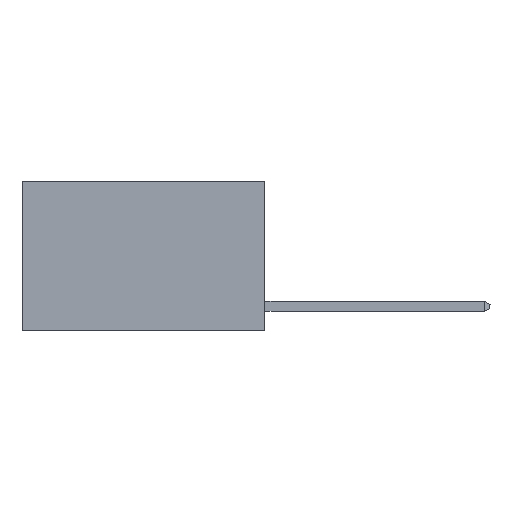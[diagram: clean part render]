
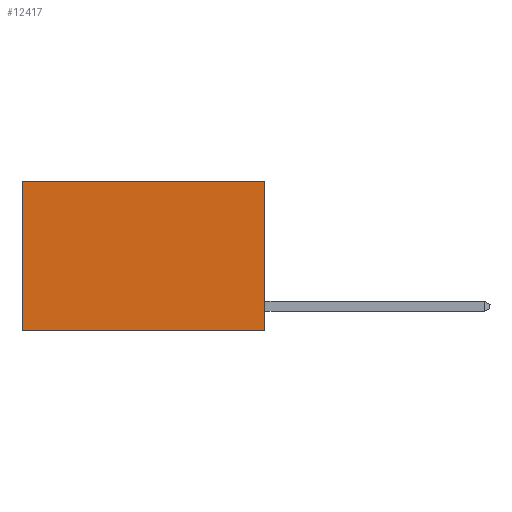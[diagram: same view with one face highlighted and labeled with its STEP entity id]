
A CAD part, left-side view. The second image highlights one B-rep face of the part: STEP entity #12417.
In plain terms, the highlighted planar face has unit normal (-1, 0, 0).
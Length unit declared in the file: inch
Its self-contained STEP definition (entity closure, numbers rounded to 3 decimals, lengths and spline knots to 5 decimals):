
#663 = CARTESIAN_POINT ( 'NONE',  ( 0.2625, 0.6, 0. ) ) ;
#1019 = CARTESIAN_POINT ( 'NONE',  ( 0.2625, 0., 0. ) ) ;
#3000 = DIRECTION ( 'NONE',  ( 0., 1., 0. ) ) ;
#4520 = CARTESIAN_POINT ( 'NONE',  ( 0.2625, 0.6, 0. ) ) ;
#4932 = ORIENTED_EDGE ( 'NONE', *, *, #5893, .F. ) ;
#5893 = EDGE_CURVE ( 'NONE', #20330, #10267, #9014, .T. ) ;
#6790 = CARTESIAN_POINT ( 'NONE',  ( 0.2625, 0.6, -0.37 ) ) ;
#6966 = DIRECTION ( 'NONE',  ( 0., 1., 0. ) ) ;
#7016 = EDGE_LOOP ( 'NONE', ( #21940, #12487, #4932, #16918 ) ) ;
#7241 = PLANE ( 'NONE',  #24932 ) ;
#7318 = DIRECTION ( 'NONE',  ( 1., 0., 0. ) ) ;
#9014 = LINE ( 'NONE', #9641, #23348 ) ;
#9641 = CARTESIAN_POINT ( 'NONE',  ( 0.2625, 0., 0. ) ) ;
#10267 = VERTEX_POINT ( 'NONE', #14692 ) ;
#10447 = LINE ( 'NONE', #4520, #14331 ) ;
#11638 = LINE ( 'NONE', #22583, #16205 ) ;
#12000 = LINE ( 'NONE', #1019, #21722 ) ;
#12280 = FACE_OUTER_BOUND ( 'NONE', #7016, .T. ) ;
#12417 = ADVANCED_FACE ( 'NONE', ( #12280 ), #7241, .F. ) ;
#12487 = ORIENTED_EDGE ( 'NONE', *, *, #14634, .F. ) ;
#12838 = EDGE_CURVE ( 'NONE', #20330, #20170, #12000, .T. ) ;
#13375 = EDGE_CURVE ( 'NONE', #20170, #23621, #10447, .T. ) ;
#14328 = DIRECTION ( 'NONE',  ( 0., 0., -1. ) ) ;
#14331 = VECTOR ( 'NONE', #14328, 39.37008 ) ;
#14634 = EDGE_CURVE ( 'NONE', #10267, #23621, #11638, .T. ) ;
#14692 = CARTESIAN_POINT ( 'NONE',  ( 0.2625, 0., -0.37 ) ) ;
#15136 = CARTESIAN_POINT ( 'NONE',  ( 0.2625, 0., 0. ) ) ;
#16205 = VECTOR ( 'NONE', #6966, 39.37008 ) ;
#16918 = ORIENTED_EDGE ( 'NONE', *, *, #12838, .T. ) ;
#17469 = DIRECTION ( 'NONE',  ( 0., 0., -1. ) ) ;
#18801 = CARTESIAN_POINT ( 'NONE',  ( 0.2625, 0., 0. ) ) ;
#20170 = VERTEX_POINT ( 'NONE', #663 ) ;
#20330 = VERTEX_POINT ( 'NONE', #18801 ) ;
#20989 = DIRECTION ( 'NONE',  ( 0., 0., -1. ) ) ;
#21722 = VECTOR ( 'NONE', #3000, 39.37008 ) ;
#21940 = ORIENTED_EDGE ( 'NONE', *, *, #13375, .T. ) ;
#22583 = CARTESIAN_POINT ( 'NONE',  ( 0.2625, 0., -0.37 ) ) ;
#23348 = VECTOR ( 'NONE', #17469, 39.37008 ) ;
#23621 = VERTEX_POINT ( 'NONE', #6790 ) ;
#24932 = AXIS2_PLACEMENT_3D ( 'NONE', #15136, #7318, #20989 ) ;
